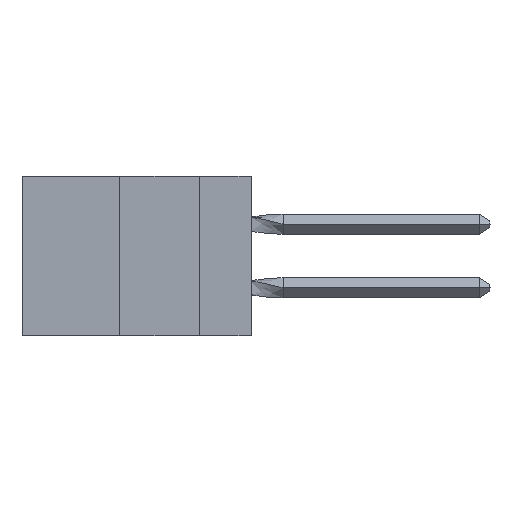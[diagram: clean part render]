
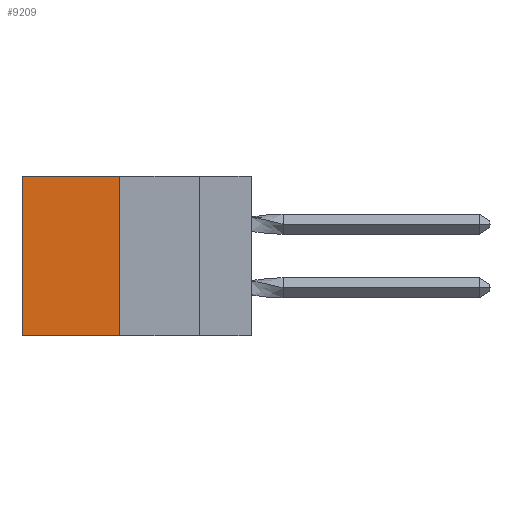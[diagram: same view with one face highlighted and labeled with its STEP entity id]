
A CAD part, left-side view. The second image highlights one B-rep face of the part: STEP entity #9209.
In plain terms, the highlighted planar face has unit normal (-1, 0, 0).
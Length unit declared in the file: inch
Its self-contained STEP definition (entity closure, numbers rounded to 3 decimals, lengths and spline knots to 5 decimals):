
#353 = LINE ( 'NONE', #7286, #4971 ) ;
#868 = PLANE ( 'NONE',  #6995 ) ;
#1607 = EDGE_CURVE ( 'NONE', #4760, #15215, #16098, .T. ) ;
#1618 = EDGE_LOOP ( 'NONE', ( #9037, #6603, #4399, #14929 ) ) ;
#2020 = DIRECTION ( 'NONE',  ( 0., 0., -1. ) ) ;
#4399 = ORIENTED_EDGE ( 'NONE', *, *, #11870, .F. ) ;
#4760 = VERTEX_POINT ( 'NONE', #14048 ) ;
#4971 = VECTOR ( 'NONE', #12504, 39.37008 ) ;
#5103 = EDGE_CURVE ( 'NONE', #15215, #6368, #353, .T. ) ;
#5357 = LINE ( 'NONE', #9835, #9992 ) ;
#6038 = CARTESIAN_POINT ( 'NONE',  ( 0.305, 0.72, 0. ) ) ;
#6273 = VECTOR ( 'NONE', #11633, 39.37008 ) ;
#6368 = VERTEX_POINT ( 'NONE', #8140 ) ;
#6470 = VECTOR ( 'NONE', #16553, 39.37008 ) ;
#6603 = ORIENTED_EDGE ( 'NONE', *, *, #8154, .F. ) ;
#6707 = FACE_OUTER_BOUND ( 'NONE', #1618, .T. ) ;
#6776 = CARTESIAN_POINT ( 'NONE',  ( 0.305, 0.413, -0.5 ) ) ;
#6995 = AXIS2_PLACEMENT_3D ( 'NONE', #13868, #8663, #15085 ) ;
#7286 = CARTESIAN_POINT ( 'NONE',  ( 0.305, 0.72, -0.5 ) ) ;
#7677 = CARTESIAN_POINT ( 'NONE',  ( 0.305, 0.413, 0. ) ) ;
#8140 = CARTESIAN_POINT ( 'NONE',  ( 0.305, 0.72, -0.5 ) ) ;
#8154 = EDGE_CURVE ( 'NONE', #15030, #6368, #13708, .T. ) ;
#8663 = DIRECTION ( 'NONE',  ( 1., 0., 0. ) ) ;
#9037 = ORIENTED_EDGE ( 'NONE', *, *, #5103, .T. ) ;
#9209 = ADVANCED_FACE ( 'NONE', ( #6707 ), #868, .F. ) ;
#9835 = CARTESIAN_POINT ( 'NONE',  ( 0.305, 0.413, -0.5 ) ) ;
#9992 = VECTOR ( 'NONE', #2020, 39.37008 ) ;
#11444 = CARTESIAN_POINT ( 'NONE',  ( 0.305, 0.413, -0.5 ) ) ;
#11633 = DIRECTION ( 'NONE',  ( 0., 1., 0. ) ) ;
#11870 = EDGE_CURVE ( 'NONE', #4760, #15030, #5357, .T. ) ;
#12504 = DIRECTION ( 'NONE',  ( 0., 0., -1. ) ) ;
#13708 = LINE ( 'NONE', #11444, #6470 ) ;
#13868 = CARTESIAN_POINT ( 'NONE',  ( 0.305, 0.413, -0.5 ) ) ;
#14048 = CARTESIAN_POINT ( 'NONE',  ( 0.305, 0.413, 0. ) ) ;
#14929 = ORIENTED_EDGE ( 'NONE', *, *, #1607, .T. ) ;
#15030 = VERTEX_POINT ( 'NONE', #6776 ) ;
#15085 = DIRECTION ( 'NONE',  ( 0., 0., -1. ) ) ;
#15215 = VERTEX_POINT ( 'NONE', #6038 ) ;
#16098 = LINE ( 'NONE', #7677, #6273 ) ;
#16553 = DIRECTION ( 'NONE',  ( 0., 1., 0. ) ) ;
